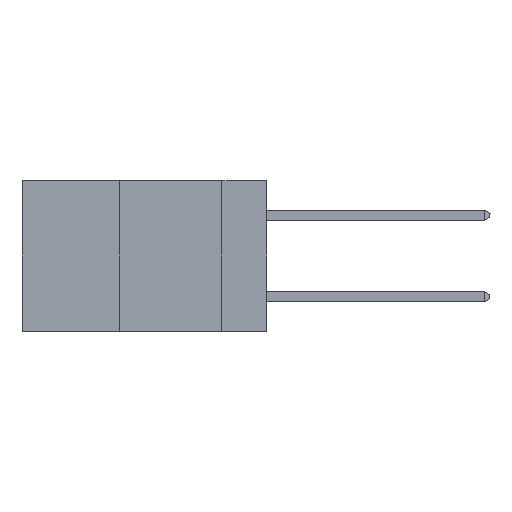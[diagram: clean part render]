
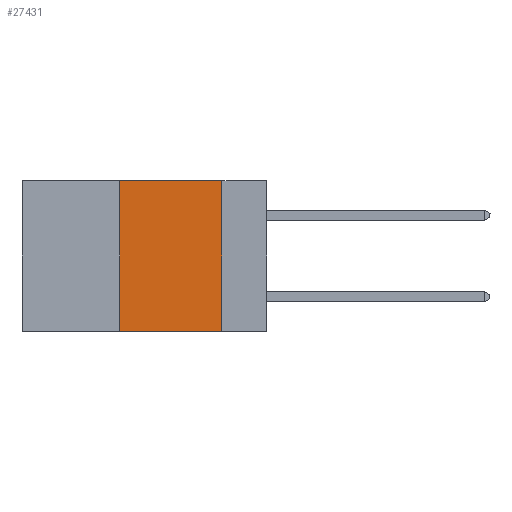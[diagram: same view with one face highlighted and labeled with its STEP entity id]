
A CAD part, left-side view. The second image highlights one B-rep face of the part: STEP entity #27431.
In plain terms, the highlighted planar face has unit normal (-1, 0, 0).
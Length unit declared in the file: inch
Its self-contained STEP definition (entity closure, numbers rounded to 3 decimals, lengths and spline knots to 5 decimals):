
#2935 = ORIENTED_EDGE ( 'NONE', *, *, #34248, .T. ) ;
#4682 = VERTEX_POINT ( 'NONE', #18266 ) ;
#5300 = LINE ( 'NONE', #44627, #37765 ) ;
#5676 = EDGE_LOOP ( 'NONE', ( #17149, #7971, #16190, #2935 ) ) ;
#7971 = ORIENTED_EDGE ( 'NONE', *, *, #42108, .F. ) ;
#9703 = DIRECTION ( 'NONE',  ( 0., -1., 0. ) ) ;
#10239 = LINE ( 'NONE', #34215, #43730 ) ;
#16190 = ORIENTED_EDGE ( 'NONE', *, *, #28620, .F. ) ;
#16237 = DIRECTION ( 'NONE',  ( 0., 0., -1. ) ) ;
#16861 = CARTESIAN_POINT ( 'NONE',  ( 0., 0.11, 0. ) ) ;
#17149 = ORIENTED_EDGE ( 'NONE', *, *, #27571, .F. ) ;
#18266 = CARTESIAN_POINT ( 'NONE',  ( 0., 0.11, -0.37 ) ) ;
#18910 = VECTOR ( 'NONE', #9703, 39.37008 ) ;
#19899 = LINE ( 'NONE', #28688, #26373 ) ;
#21531 = VERTEX_POINT ( 'NONE', #25323 ) ;
#22797 = CARTESIAN_POINT ( 'NONE',  ( 0., 0.36, -0.37 ) ) ;
#23080 = CARTESIAN_POINT ( 'NONE',  ( 0., 0.6, 0. ) ) ;
#24287 = AXIS2_PLACEMENT_3D ( 'NONE', #23080, #39805, #16237 ) ;
#25323 = CARTESIAN_POINT ( 'NONE',  ( 0., 0.36, 0. ) ) ;
#26064 = PLANE ( 'NONE',  #24287 ) ;
#26373 = VECTOR ( 'NONE', #35639, 39.37008 ) ;
#27431 = ADVANCED_FACE ( 'NONE', ( #36216 ), #26064, .F. ) ;
#27567 = LINE ( 'NONE', #43838, #18910 ) ;
#27571 = EDGE_CURVE ( 'NONE', #39828, #4682, #10239, .T. ) ;
#28620 = EDGE_CURVE ( 'NONE', #34022, #21531, #19899, .T. ) ;
#28688 = CARTESIAN_POINT ( 'NONE',  ( 0., 0.36, 0. ) ) ;
#34022 = VERTEX_POINT ( 'NONE', #22797 ) ;
#34064 = DIRECTION ( 'NONE',  ( 0., 0., -1. ) ) ;
#34215 = CARTESIAN_POINT ( 'NONE',  ( 0., 0.11, 0. ) ) ;
#34248 = EDGE_CURVE ( 'NONE', #34022, #4682, #5300, .T. ) ;
#35639 = DIRECTION ( 'NONE',  ( 0., 0., 1. ) ) ;
#36216 = FACE_OUTER_BOUND ( 'NONE', #5676, .T. ) ;
#37765 = VECTOR ( 'NONE', #41005, 39.37008 ) ;
#39805 = DIRECTION ( 'NONE',  ( 1., 0., 0. ) ) ;
#39828 = VERTEX_POINT ( 'NONE', #16861 ) ;
#41005 = DIRECTION ( 'NONE',  ( 0., -1., 0. ) ) ;
#42108 = EDGE_CURVE ( 'NONE', #21531, #39828, #27567, .T. ) ;
#43730 = VECTOR ( 'NONE', #34064, 39.37008 ) ;
#43838 = CARTESIAN_POINT ( 'NONE',  ( 0., 0.6, 0. ) ) ;
#44627 = CARTESIAN_POINT ( 'NONE',  ( 0., 0.6, -0.37 ) ) ;
